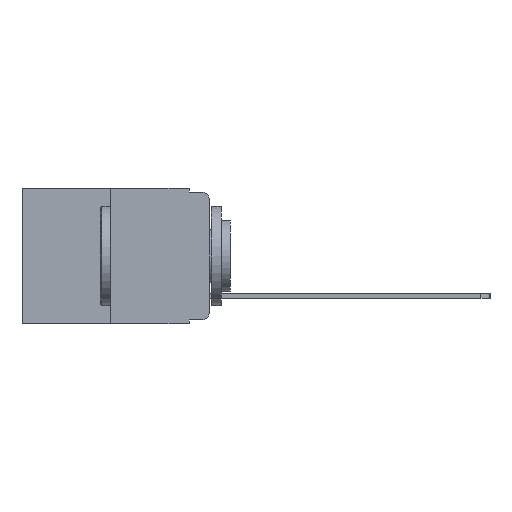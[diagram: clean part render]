
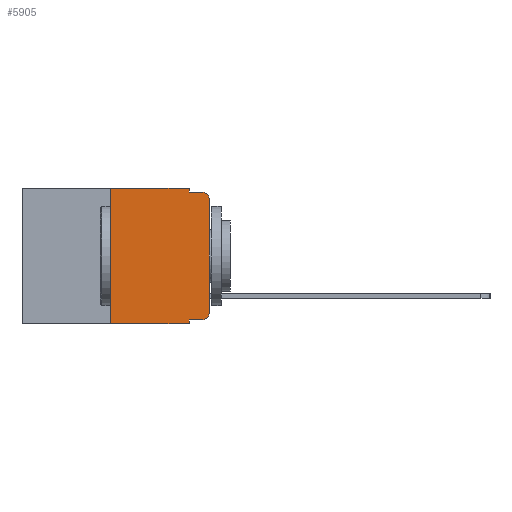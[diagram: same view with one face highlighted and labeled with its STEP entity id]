
A CAD part, left-side view. The second image highlights one B-rep face of the part: STEP entity #5905.
In plain terms, the highlighted planar face has unit normal (-1, 0, 0).
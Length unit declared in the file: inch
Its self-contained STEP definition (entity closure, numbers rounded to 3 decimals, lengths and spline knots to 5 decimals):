
#4 = DIRECTION ( 'NONE',  ( -1., 0., 0. ) ) ;
#203 = LINE ( 'NONE', #17046, #8203 ) ;
#336 = DIRECTION ( 'NONE',  ( 0., -1., 0. ) ) ;
#774 = CIRCLE ( 'NONE', #8637, 0.02 ) ;
#1097 = ORIENTED_EDGE ( 'NONE', *, *, #5687, .T. ) ;
#1121 = LINE ( 'NONE', #6381, #11431 ) ;
#1572 = CARTESIAN_POINT ( 'NONE',  ( 0., 0., -0.313 ) ) ;
#1584 = DIRECTION ( 'NONE',  ( 0., 0., 1. ) ) ;
#1896 = LINE ( 'NONE', #4726, #15535 ) ;
#1938 = ORIENTED_EDGE ( 'NONE', *, *, #11345, .T. ) ;
#2314 = VERTEX_POINT ( 'NONE', #8961 ) ;
#2322 = LINE ( 'NONE', #14584, #9089 ) ;
#2677 = DIRECTION ( 'NONE',  ( 0., -1., 0. ) ) ;
#2907 = VERTEX_POINT ( 'NONE', #15817 ) ;
#2926 = VERTEX_POINT ( 'NONE', #16844 ) ;
#2971 = EDGE_CURVE ( 'NONE', #2907, #8752, #203, .T. ) ;
#3683 = CARTESIAN_POINT ( 'NONE',  ( 0., 0.02, -0.313 ) ) ;
#3860 = VERTEX_POINT ( 'NONE', #6798 ) ;
#4140 = CARTESIAN_POINT ( 'NONE',  ( 0., 0.051, -0.343 ) ) ;
#4192 = CARTESIAN_POINT ( 'NONE',  ( 0., 0.051, -0.333 ) ) ;
#4212 = DIRECTION ( 'NONE',  ( 0., 0., -1. ) ) ;
#4216 = VECTOR ( 'NONE', #4212, 39.37008 ) ;
#4419 = AXIS2_PLACEMENT_3D ( 'NONE', #16296, #13794, #5871 ) ;
#4485 = VERTEX_POINT ( 'NONE', #1572 ) ;
#4644 = LINE ( 'NONE', #12236, #4216 ) ;
#4726 = CARTESIAN_POINT ( 'NONE',  ( 0., 0., 0. ) ) ;
#5060 = DIRECTION ( 'NONE',  ( 0., 0., -1. ) ) ;
#5533 = LINE ( 'NONE', #16408, #15992 ) ;
#5687 = EDGE_CURVE ( 'NONE', #3860, #8752, #14479, .T. ) ;
#5835 = EDGE_LOOP ( 'NONE', ( #7834, #1097, #11794, #15194, #12196, #15575, #1938, #12594, #15965, #9526 ) ) ;
#5871 = DIRECTION ( 'NONE',  ( 0., 0., -1. ) ) ;
#5905 = ADVANCED_FACE ( 'NONE', ( #12773 ), #11234, .F. ) ;
#6316 = VERTEX_POINT ( 'NONE', #4192 ) ;
#6381 = CARTESIAN_POINT ( 'NONE',  ( 0., 0.051, -0.333 ) ) ;
#6580 = AXIS2_PLACEMENT_3D ( 'NONE', #8065, #4, #9422 ) ;
#6600 = EDGE_CURVE ( 'NONE', #4485, #3860, #1896, .T. ) ;
#6798 = CARTESIAN_POINT ( 'NONE',  ( 0., 0., -0.03 ) ) ;
#7001 = CARTESIAN_POINT ( 'NONE',  ( 0., 0.051, 0. ) ) ;
#7834 = ORIENTED_EDGE ( 'NONE', *, *, #6600, .T. ) ;
#8065 = CARTESIAN_POINT ( 'NONE',  ( 0., 0.02, -0.03 ) ) ;
#8203 = VECTOR ( 'NONE', #14968, 39.37008 ) ;
#8637 = AXIS2_PLACEMENT_3D ( 'NONE', #3683, #13028, #5060 ) ;
#8652 = DIRECTION ( 'NONE',  ( 0., 0., -1. ) ) ;
#8736 = EDGE_CURVE ( 'NONE', #2926, #4485, #774, .T. ) ;
#8752 = VERTEX_POINT ( 'NONE', #8775 ) ;
#8775 = CARTESIAN_POINT ( 'NONE',  ( 0., 0.02, -0.01 ) ) ;
#8914 = VERTEX_POINT ( 'NONE', #4140 ) ;
#8961 = CARTESIAN_POINT ( 'NONE',  ( 0., 0.25, -0.343 ) ) ;
#9089 = VECTOR ( 'NONE', #2677, 39.37008 ) ;
#9422 = DIRECTION ( 'NONE',  ( 0., 0., -1. ) ) ;
#9526 = ORIENTED_EDGE ( 'NONE', *, *, #8736, .T. ) ;
#9733 = CARTESIAN_POINT ( 'NONE',  ( 0., 0.25, 0. ) ) ;
#10551 = EDGE_CURVE ( 'NONE', #6316, #2926, #1121, .T. ) ;
#10569 = LINE ( 'NONE', #16163, #13586 ) ;
#11000 = CARTESIAN_POINT ( 'NONE',  ( 0., 0.25, 0. ) ) ;
#11234 = PLANE ( 'NONE',  #4419 ) ;
#11345 = EDGE_CURVE ( 'NONE', #2314, #8914, #2322, .T. ) ;
#11431 = VECTOR ( 'NONE', #14275, 39.37008 ) ;
#11441 = EDGE_CURVE ( 'NONE', #6316, #8914, #4644, .T. ) ;
#11507 = DIRECTION ( 'NONE',  ( 0., 0., 1. ) ) ;
#11514 = LINE ( 'NONE', #11000, #14092 ) ;
#11794 = ORIENTED_EDGE ( 'NONE', *, *, #2971, .F. ) ;
#12093 = EDGE_CURVE ( 'NONE', #15149, #16978, #10569, .T. ) ;
#12196 = ORIENTED_EDGE ( 'NONE', *, *, #12093, .F. ) ;
#12236 = CARTESIAN_POINT ( 'NONE',  ( 0., 0.051, 0. ) ) ;
#12594 = ORIENTED_EDGE ( 'NONE', *, *, #11441, .F. ) ;
#12773 = FACE_OUTER_BOUND ( 'NONE', #5835, .T. ) ;
#13028 = DIRECTION ( 'NONE',  ( -1., 0., 0. ) ) ;
#13586 = VECTOR ( 'NONE', #336, 39.37008 ) ;
#13794 = DIRECTION ( 'NONE',  ( 1., 0., 0. ) ) ;
#13997 = EDGE_CURVE ( 'NONE', #2314, #15149, #11514, .T. ) ;
#14092 = VECTOR ( 'NONE', #1584, 39.37008 ) ;
#14275 = DIRECTION ( 'NONE',  ( 0., -1., 0. ) ) ;
#14479 = CIRCLE ( 'NONE', #6580, 0.02 ) ;
#14584 = CARTESIAN_POINT ( 'NONE',  ( 0., 0.473, -0.343 ) ) ;
#14968 = DIRECTION ( 'NONE',  ( 0., -1., 0. ) ) ;
#15149 = VERTEX_POINT ( 'NONE', #9733 ) ;
#15194 = ORIENTED_EDGE ( 'NONE', *, *, #16531, .F. ) ;
#15535 = VECTOR ( 'NONE', #11507, 39.37008 ) ;
#15575 = ORIENTED_EDGE ( 'NONE', *, *, #13997, .F. ) ;
#15817 = CARTESIAN_POINT ( 'NONE',  ( 0., 0.051, -0.01 ) ) ;
#15965 = ORIENTED_EDGE ( 'NONE', *, *, #10551, .T. ) ;
#15992 = VECTOR ( 'NONE', #8652, 39.37008 ) ;
#16163 = CARTESIAN_POINT ( 'NONE',  ( 0., 0.473, 0. ) ) ;
#16296 = CARTESIAN_POINT ( 'NONE',  ( 0., 0.473, 0. ) ) ;
#16408 = CARTESIAN_POINT ( 'NONE',  ( 0., 0.051, 0. ) ) ;
#16531 = EDGE_CURVE ( 'NONE', #16978, #2907, #5533, .T. ) ;
#16844 = CARTESIAN_POINT ( 'NONE',  ( 0., 0.02, -0.333 ) ) ;
#16978 = VERTEX_POINT ( 'NONE', #7001 ) ;
#17046 = CARTESIAN_POINT ( 'NONE',  ( 0., 0.051, -0.01 ) ) ;
